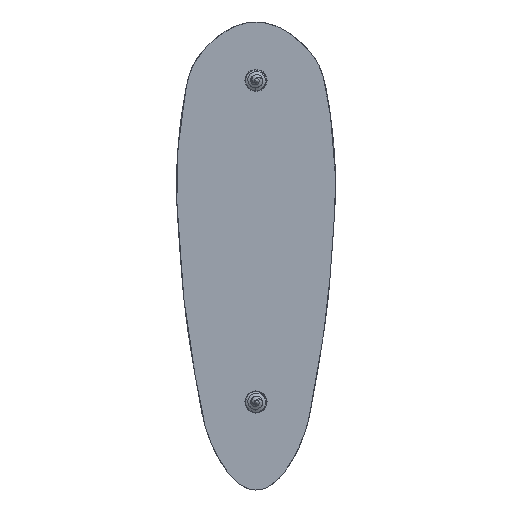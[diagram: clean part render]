
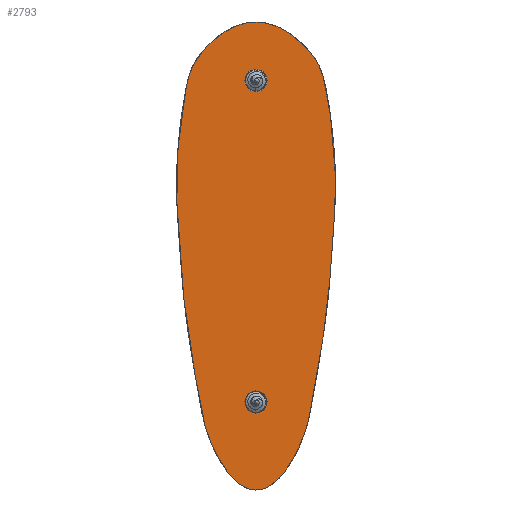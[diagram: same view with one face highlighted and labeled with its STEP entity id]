
A CAD part, front view. The second image highlights one B-rep face of the part: STEP entity #2793.
In plain terms, the highlighted planar face has unit normal (0, -1, 0).
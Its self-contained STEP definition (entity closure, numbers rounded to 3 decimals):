
#55=PLANE('',#3042);
#75=(
BOUNDED_CURVE()
B_SPLINE_CURVE(5,(#8498,#8499,#8500,#8501,#8502,#8503,#8504,#8505,#8506,
#8507,#8508,#8509,#8510,#8511,#8512,#8513,#8514,#8515,#8516,#8517,#8518,
#8519,#8520,#8521,#8522,#8523,#8524,#8525,#8526,#8527,#8528,#8529,#8530,
#8531,#8532,#8533,#8534,#8535,#8536,#8537,#8538,#8539,#8540,#8541,#8542,
#8543,#8544,#8545,#8546,#8547,#8548,#8549,#8550,#8551,#8552,#8553,#8554,
#8555,#8556,#8557,#8558,#8559,#8560,#8561,#8562,#8563,#8564,#8565,#8566,
#8567,#8568,#8569,#8570,#8571,#8572,#8573,#8574,#8575,#8576,#8577,#8578,
#8579,#8580,#8581,#8582),.UNSPECIFIED.,.T.,.F.)
B_SPLINE_CURVE_WITH_KNOTS((6,1,1,1,1,1,1,1,1,1,1,1,1,1,1,1,1,1,1,1,1,1,
1,1,1,1,1,1,1,1,1,1,1,1,1,1,1,1,1,1,1,1,1,1,1,1,1,1,1,1,1,1,1,1,1,1,1,1,
1,1,1,1,1,1,1,1,1,1,1,1,1,1,1,1,1,1,1,1,1,1,6),(0.,0.013,0.025,0.038,
0.05,0.063,0.075,0.088,0.1,0.113,0.125,0.138,0.15,0.163,0.175,0.188,
0.2,0.213,0.225,0.238,0.25,0.263,0.275,0.288,0.3,0.313,0.325,0.338,
0.35,0.363,0.375,0.388,0.4,0.413,0.425,0.438,0.45,0.463,0.475,0.488,
0.5,0.513,0.525,0.538,0.55,0.563,0.575,0.588,0.6,0.613,0.625,0.638,
0.65,0.663,0.675,0.688,0.7,0.712,0.725,0.737,
0.75,0.762,0.775,0.787,
0.8,0.812,0.825,0.837,
0.85,0.862,0.875,0.887,
0.9,0.912,0.925,0.937,
0.95,0.962,0.975,0.987,
1.),.UNSPECIFIED.)
CURVE()
GEOMETRIC_REPRESENTATION_ITEM()
RATIONAL_B_SPLINE_CURVE((1.,1.,1.,1.,1.,1.,1.,1.,1.,1.,1.,1.,1.,1.,1.,1.,
1.,1.,1.,1.,1.,1.,1.,1.,1.,1.,1.,1.,1.,1.,1.,1.,1.,1.,1.,1.,1.,1.,1.,1.,
1.,1.,1.,1.,1.,1.,1.,1.,1.,1.,1.,1.,1.,1.,1.,1.,1.,1.,1.,1.,1.,1.,1.,1.,
1.,1.,1.,1.,1.,1.,1.,1.,1.,1.,1.,1.,1.,1.,1.,1.,1.,1.,1.,1.,1.))
REPRESENTATION_ITEM('')
);
#128=FACE_BOUND('',#462,.T.);
#129=FACE_BOUND('',#463,.T.);
#270=FACE_OUTER_BOUND('',#461,.T.);
#461=EDGE_LOOP('',(#2120));
#462=EDGE_LOOP('',(#2121));
#463=EDGE_LOOP('',(#2122));
#787=CIRCLE('',#3043,2.6);
#788=CIRCLE('',#3044,2.6);
#1254=VERTEX_POINT('',#8497);
#1255=VERTEX_POINT('',#8583);
#1256=VERTEX_POINT('',#8585);
#1555=EDGE_CURVE('',#1254,#1254,#75,.T.);
#1556=EDGE_CURVE('',#1255,#1255,#787,.F.);
#1557=EDGE_CURVE('',#1256,#1256,#788,.F.);
#2120=ORIENTED_EDGE('',*,*,#1555,.T.);
#2121=ORIENTED_EDGE('',*,*,#1556,.F.);
#2122=ORIENTED_EDGE('',*,*,#1557,.F.);
#2793=ADVANCED_FACE('',(#270,#128,#129),#55,.F.);
#3042=AXIS2_PLACEMENT_3D('',#8496,#3484,#3485);
#3043=AXIS2_PLACEMENT_3D('',#8584,#3486,#3487);
#3044=AXIS2_PLACEMENT_3D('',#8586,#3488,#3489);
#3484=DIRECTION('center_axis',(0.,1.,0.));
#3485=DIRECTION('ref_axis',(1.,0.,0.));
#3486=DIRECTION('center_axis',(0.,1.,0.));
#3487=DIRECTION('ref_axis',(1.,0.,0.));
#3488=DIRECTION('center_axis',(0.,1.,0.));
#3489=DIRECTION('ref_axis',(1.,0.,0.));
#8496=CARTESIAN_POINT('Origin',(0.,0.,-41.337));
#8497=CARTESIAN_POINT('',(0.,0.,13.7));
#8498=CARTESIAN_POINT('Ctrl Pts',(0.,0.,13.7));
#8499=CARTESIAN_POINT('Ctrl Pts',(-0.627,0.,13.7));
#8500=CARTESIAN_POINT('Ctrl Pts',(-1.88,0.,13.614));
#8501=CARTESIAN_POINT('Ctrl Pts',(-3.744,0.,13.226));
#8502=CARTESIAN_POINT('Ctrl Pts',(-6.131,0.,12.238));
#8503=CARTESIAN_POINT('Ctrl Pts',(-8.806,0.,10.478));
#8504=CARTESIAN_POINT('Ctrl Pts',(-11.059,0.,8.498));
#8505=CARTESIAN_POINT('Ctrl Pts',(-12.833,0.,6.557));
#8506=CARTESIAN_POINT('Ctrl Pts',(-14.138,0.,4.765));
#8507=CARTESIAN_POINT('Ctrl Pts',(-15.069,0.,3.014));
#8508=CARTESIAN_POINT('Ctrl Pts',(-15.755,0.,1.093));
#8509=CARTESIAN_POINT('Ctrl Pts',(-16.324,0.,-1.218));
#8510=CARTESIAN_POINT('Ctrl Pts',(-16.856,0.,-4.027));
#8511=CARTESIAN_POINT('Ctrl Pts',(-17.367,0.,-7.305));
#8512=CARTESIAN_POINT('Ctrl Pts',(-17.841,0.,-10.943));
#8513=CARTESIAN_POINT('Ctrl Pts',(-18.24,0.,-14.782));
#8514=CARTESIAN_POINT('Ctrl Pts',(-18.523,0.,-18.653));
#8515=CARTESIAN_POINT('Ctrl Pts',(-18.663,0.,-22.416));
#8516=CARTESIAN_POINT('Ctrl Pts',(-18.664,0.,-26.));
#8517=CARTESIAN_POINT('Ctrl Pts',(-18.553,0.,-29.388));
#8518=CARTESIAN_POINT('Ctrl Pts',(-18.367,0.,-32.609));
#8519=CARTESIAN_POINT('Ctrl Pts',(-18.146,0.,-35.718));
#8520=CARTESIAN_POINT('Ctrl Pts',(-17.92,0.,-38.788));
#8521=CARTESIAN_POINT('Ctrl Pts',(-17.698,0.,-41.892));
#8522=CARTESIAN_POINT('Ctrl Pts',(-17.464,0.,-45.095));
#8523=CARTESIAN_POINT('Ctrl Pts',(-17.191,0.,-48.443));
#8524=CARTESIAN_POINT('Ctrl Pts',(-16.85,0.,-51.956));
#8525=CARTESIAN_POINT('Ctrl Pts',(-16.417,0.,-55.624));
#8526=CARTESIAN_POINT('Ctrl Pts',(-15.889,0.,-59.394));
#8527=CARTESIAN_POINT('Ctrl Pts',(-15.293,0.,-63.162));
#8528=CARTESIAN_POINT('Ctrl Pts',(-14.676,0.,-66.794));
#8529=CARTESIAN_POINT('Ctrl Pts',(-14.085,0.,-70.163));
#8530=CARTESIAN_POINT('Ctrl Pts',(-13.557,0.,-73.178));
#8531=CARTESIAN_POINT('Ctrl Pts',(-13.097,0.,-75.815));
#8532=CARTESIAN_POINT('Ctrl Pts',(-12.664,0.,-78.152));
#8533=CARTESIAN_POINT('Ctrl Pts',(-12.157,0.,-80.391));
#8534=CARTESIAN_POINT('Ctrl Pts',(-11.452,0.,-82.754));
#8535=CARTESIAN_POINT('Ctrl Pts',(-10.432,0.,-85.4));
#8536=CARTESIAN_POINT('Ctrl Pts',(-9.015,0.,-88.334));
#8537=CARTESIAN_POINT('Ctrl Pts',(-7.193,0.,-91.305));
#8538=CARTESIAN_POINT('Ctrl Pts',(-5.015,0.,-93.912));
#8539=CARTESIAN_POINT('Ctrl Pts',(-2.577,0.,-95.72));
#8540=CARTESIAN_POINT('Ctrl Pts',(0.,0.,-96.375));
#8541=CARTESIAN_POINT('Ctrl Pts',(2.577,0.,-95.72));
#8542=CARTESIAN_POINT('Ctrl Pts',(5.015,0.,-93.912));
#8543=CARTESIAN_POINT('Ctrl Pts',(7.193,0.,-91.305));
#8544=CARTESIAN_POINT('Ctrl Pts',(9.015,0.,-88.334));
#8545=CARTESIAN_POINT('Ctrl Pts',(10.432,0.,-85.4));
#8546=CARTESIAN_POINT('Ctrl Pts',(11.452,0.,-82.754));
#8547=CARTESIAN_POINT('Ctrl Pts',(12.157,0.,-80.391));
#8548=CARTESIAN_POINT('Ctrl Pts',(12.664,0.,-78.152));
#8549=CARTESIAN_POINT('Ctrl Pts',(13.097,0.,-75.815));
#8550=CARTESIAN_POINT('Ctrl Pts',(13.557,0.,-73.178));
#8551=CARTESIAN_POINT('Ctrl Pts',(14.085,0.,-70.163));
#8552=CARTESIAN_POINT('Ctrl Pts',(14.676,0.,-66.794));
#8553=CARTESIAN_POINT('Ctrl Pts',(15.293,0.,-63.162));
#8554=CARTESIAN_POINT('Ctrl Pts',(15.889,0.,-59.394));
#8555=CARTESIAN_POINT('Ctrl Pts',(16.417,0.,-55.624));
#8556=CARTESIAN_POINT('Ctrl Pts',(16.85,0.,-51.956));
#8557=CARTESIAN_POINT('Ctrl Pts',(17.191,0.,-48.443));
#8558=CARTESIAN_POINT('Ctrl Pts',(17.464,0.,-45.095));
#8559=CARTESIAN_POINT('Ctrl Pts',(17.698,0.,-41.892));
#8560=CARTESIAN_POINT('Ctrl Pts',(17.92,0.,-38.788));
#8561=CARTESIAN_POINT('Ctrl Pts',(18.146,0.,-35.718));
#8562=CARTESIAN_POINT('Ctrl Pts',(18.367,0.,-32.609));
#8563=CARTESIAN_POINT('Ctrl Pts',(18.553,0.,-29.388));
#8564=CARTESIAN_POINT('Ctrl Pts',(18.664,0.,-26.));
#8565=CARTESIAN_POINT('Ctrl Pts',(18.663,0.,-22.416));
#8566=CARTESIAN_POINT('Ctrl Pts',(18.523,0.,-18.653));
#8567=CARTESIAN_POINT('Ctrl Pts',(18.24,0.,-14.782));
#8568=CARTESIAN_POINT('Ctrl Pts',(17.841,0.,-10.943));
#8569=CARTESIAN_POINT('Ctrl Pts',(17.367,0.,-7.305));
#8570=CARTESIAN_POINT('Ctrl Pts',(16.856,0.,-4.027));
#8571=CARTESIAN_POINT('Ctrl Pts',(16.324,0.,-1.218));
#8572=CARTESIAN_POINT('Ctrl Pts',(15.755,0.,1.093));
#8573=CARTESIAN_POINT('Ctrl Pts',(15.069,0.,3.014));
#8574=CARTESIAN_POINT('Ctrl Pts',(14.138,0.,4.765));
#8575=CARTESIAN_POINT('Ctrl Pts',(12.833,0.,6.557));
#8576=CARTESIAN_POINT('Ctrl Pts',(11.059,0.,8.498));
#8577=CARTESIAN_POINT('Ctrl Pts',(8.806,0.,10.478));
#8578=CARTESIAN_POINT('Ctrl Pts',(6.131,0.,12.238));
#8579=CARTESIAN_POINT('Ctrl Pts',(3.744,0.,13.226));
#8580=CARTESIAN_POINT('Ctrl Pts',(1.88,0.,13.614));
#8581=CARTESIAN_POINT('Ctrl Pts',(0.627,0.,13.7));
#8582=CARTESIAN_POINT('Ctrl Pts',(0.,0.,13.7));
#8583=CARTESIAN_POINT('',(-2.6,0.,0.));
#8584=CARTESIAN_POINT('Origin',(0.,0.,0.));
#8585=CARTESIAN_POINT('',(-2.6,0.,-75.4));
#8586=CARTESIAN_POINT('Origin',(0.,0.,-75.4));
